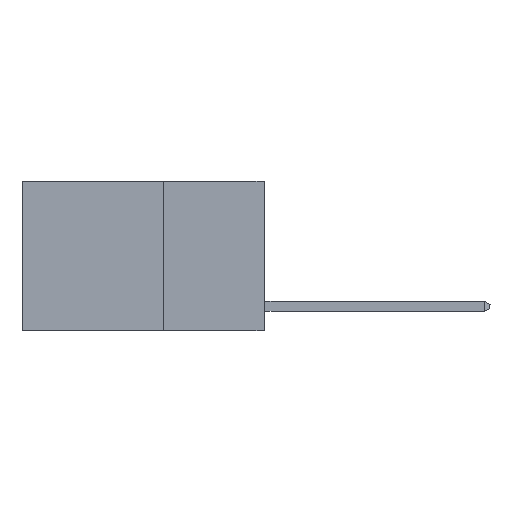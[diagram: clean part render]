
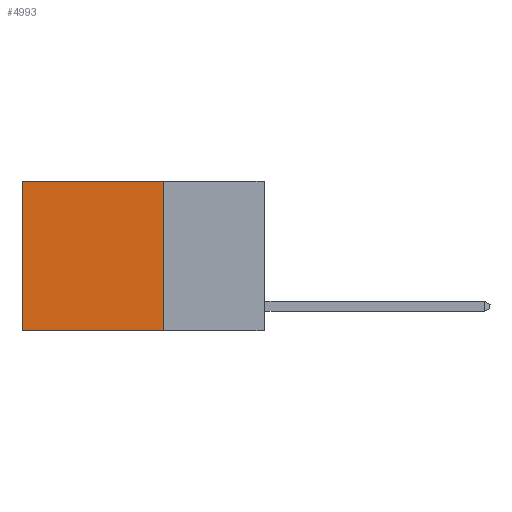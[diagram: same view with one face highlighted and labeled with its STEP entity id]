
A CAD part, left-side view. The second image highlights one B-rep face of the part: STEP entity #4993.
In plain terms, the highlighted planar face has unit normal (-1, 0, 0).
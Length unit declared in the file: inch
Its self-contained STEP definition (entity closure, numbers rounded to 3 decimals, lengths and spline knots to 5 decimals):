
#439 = CARTESIAN_POINT ( 'NONE',  ( 0.2625, 0.25, 0. ) ) ;
#1005 = VERTEX_POINT ( 'NONE', #12233 ) ;
#1704 = CARTESIAN_POINT ( 'NONE',  ( 0.2625, 0.25, 0. ) ) ;
#1708 = DIRECTION ( 'NONE',  ( 0., 1., 0. ) ) ;
#2417 = LINE ( 'NONE', #439, #11855 ) ;
#2710 = EDGE_CURVE ( 'NONE', #7595, #10328, #11857, .T. ) ;
#3390 = FACE_OUTER_BOUND ( 'NONE', #10442, .T. ) ;
#4135 = PLANE ( 'NONE',  #9812 ) ;
#4539 = ORIENTED_EDGE ( 'NONE', *, *, #7370, .T. ) ;
#4732 = CARTESIAN_POINT ( 'NONE',  ( 0.2625, 0.6, 0. ) ) ;
#4993 = ADVANCED_FACE ( 'NONE', ( #3390 ), #4135, .F. ) ;
#5140 = VECTOR ( 'NONE', #7605, 39.37008 ) ;
#5387 = DIRECTION ( 'NONE',  ( 0., 0., -1. ) ) ;
#5536 = LINE ( 'NONE', #12010, #5140 ) ;
#6001 = VECTOR ( 'NONE', #6110, 39.37008 ) ;
#6110 = DIRECTION ( 'NONE',  ( 0., 1., 0. ) ) ;
#7370 = EDGE_CURVE ( 'NONE', #1005, #13256, #2417, .T. ) ;
#7595 = VERTEX_POINT ( 'NONE', #12371 ) ;
#7605 = DIRECTION ( 'NONE',  ( 0., 0., -1. ) ) ;
#7853 = VECTOR ( 'NONE', #9092, 39.37008 ) ;
#8021 = ORIENTED_EDGE ( 'NONE', *, *, #2710, .F. ) ;
#9092 = DIRECTION ( 'NONE',  ( 0., 0., -1. ) ) ;
#9368 = EDGE_CURVE ( 'NONE', #13256, #10328, #5536, .T. ) ;
#9812 = AXIS2_PLACEMENT_3D ( 'NONE', #1704, #12028, #5387 ) ;
#10328 = VERTEX_POINT ( 'NONE', #14398 ) ;
#10442 = EDGE_LOOP ( 'NONE', ( #12872, #8021, #12094, #4539 ) ) ;
#11133 = LINE ( 'NONE', #13505, #7853 ) ;
#11855 = VECTOR ( 'NONE', #1708, 39.37008 ) ;
#11857 = LINE ( 'NONE', #12675, #6001 ) ;
#12010 = CARTESIAN_POINT ( 'NONE',  ( 0.2625, 0.6, 0. ) ) ;
#12028 = DIRECTION ( 'NONE',  ( 1., 0., 0. ) ) ;
#12094 = ORIENTED_EDGE ( 'NONE', *, *, #13130, .F. ) ;
#12233 = CARTESIAN_POINT ( 'NONE',  ( 0.2625, 0.25, 0. ) ) ;
#12371 = CARTESIAN_POINT ( 'NONE',  ( 0.2625, 0.25, -0.37 ) ) ;
#12675 = CARTESIAN_POINT ( 'NONE',  ( 0.2625, 0.25, -0.37 ) ) ;
#12872 = ORIENTED_EDGE ( 'NONE', *, *, #9368, .T. ) ;
#13130 = EDGE_CURVE ( 'NONE', #1005, #7595, #11133, .T. ) ;
#13256 = VERTEX_POINT ( 'NONE', #4732 ) ;
#13505 = CARTESIAN_POINT ( 'NONE',  ( 0.2625, 0.25, 0. ) ) ;
#14398 = CARTESIAN_POINT ( 'NONE',  ( 0.2625, 0.6, -0.37 ) ) ;
